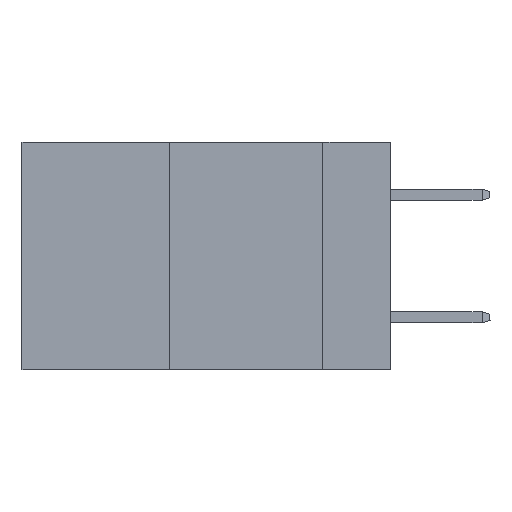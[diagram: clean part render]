
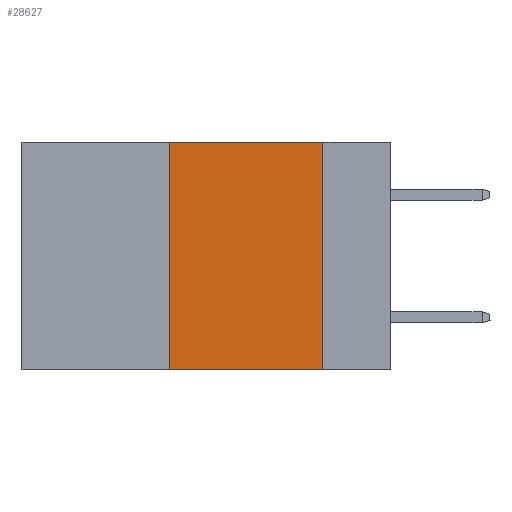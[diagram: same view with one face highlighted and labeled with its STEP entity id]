
A CAD part, left-side view. The second image highlights one B-rep face of the part: STEP entity #28627.
In plain terms, the highlighted planar face has unit normal (-1, 0, 0).
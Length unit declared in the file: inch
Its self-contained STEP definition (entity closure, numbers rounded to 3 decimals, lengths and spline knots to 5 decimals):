
#39 = DIRECTION ( 'NONE',  ( 0., -1., 0. ) ) ;
#258 = EDGE_CURVE ( 'NONE', #45079, #8509, #11743, .T. ) ;
#582 = EDGE_CURVE ( 'NONE', #22951, #24627, #32316, .T. ) ;
#1089 = VECTOR ( 'NONE', #42020, 39.37008 ) ;
#3551 = EDGE_CURVE ( 'NONE', #8509, #22951, #22784, .T. ) ;
#5698 = CARTESIAN_POINT ( 'NONE',  ( 0., 0.36, 0. ) ) ;
#6953 = CARTESIAN_POINT ( 'NONE',  ( 0., 0.6, -0.37 ) ) ;
#8509 = VERTEX_POINT ( 'NONE', #5698 ) ;
#8948 = CARTESIAN_POINT ( 'NONE',  ( 0., 0.11, -0.37 ) ) ;
#10359 = EDGE_LOOP ( 'NONE', ( #26051, #21625, #26498, #43389 ) ) ;
#11743 = LINE ( 'NONE', #31594, #1089 ) ;
#12289 = VECTOR ( 'NONE', #35083, 39.37008 ) ;
#12450 = PLANE ( 'NONE',  #37120 ) ;
#15904 = VECTOR ( 'NONE', #30992, 39.37008 ) ;
#19597 = DIRECTION ( 'NONE',  ( 0., 0., -1. ) ) ;
#21625 = ORIENTED_EDGE ( 'NONE', *, *, #3551, .F. ) ;
#21909 = LINE ( 'NONE', #6953, #28975 ) ;
#22784 = LINE ( 'NONE', #33488, #12289 ) ;
#22951 = VERTEX_POINT ( 'NONE', #27642 ) ;
#24627 = VERTEX_POINT ( 'NONE', #8948 ) ;
#26051 = ORIENTED_EDGE ( 'NONE', *, *, #582, .F. ) ;
#26498 = ORIENTED_EDGE ( 'NONE', *, *, #258, .F. ) ;
#26617 = CARTESIAN_POINT ( 'NONE',  ( 0., 0.36, -0.37 ) ) ;
#26970 = FACE_OUTER_BOUND ( 'NONE', #10359, .T. ) ;
#27344 = CARTESIAN_POINT ( 'NONE',  ( 0., 0.11, 0. ) ) ;
#27642 = CARTESIAN_POINT ( 'NONE',  ( 0., 0.11, 0. ) ) ;
#28627 = ADVANCED_FACE ( 'NONE', ( #26970 ), #12450, .F. ) ;
#28975 = VECTOR ( 'NONE', #39, 39.37008 ) ;
#30992 = DIRECTION ( 'NONE',  ( 0., 0., -1. ) ) ;
#31594 = CARTESIAN_POINT ( 'NONE',  ( 0., 0.36, 0. ) ) ;
#32316 = LINE ( 'NONE', #27344, #15904 ) ;
#33488 = CARTESIAN_POINT ( 'NONE',  ( 0., 0.6, 0. ) ) ;
#35083 = DIRECTION ( 'NONE',  ( 0., -1., 0. ) ) ;
#36882 = CARTESIAN_POINT ( 'NONE',  ( 0., 0.6, 0. ) ) ;
#37120 = AXIS2_PLACEMENT_3D ( 'NONE', #36882, #40352, #19597 ) ;
#40352 = DIRECTION ( 'NONE',  ( 1., 0., 0. ) ) ;
#40675 = EDGE_CURVE ( 'NONE', #45079, #24627, #21909, .T. ) ;
#42020 = DIRECTION ( 'NONE',  ( 0., 0., 1. ) ) ;
#43389 = ORIENTED_EDGE ( 'NONE', *, *, #40675, .T. ) ;
#45079 = VERTEX_POINT ( 'NONE', #26617 ) ;
